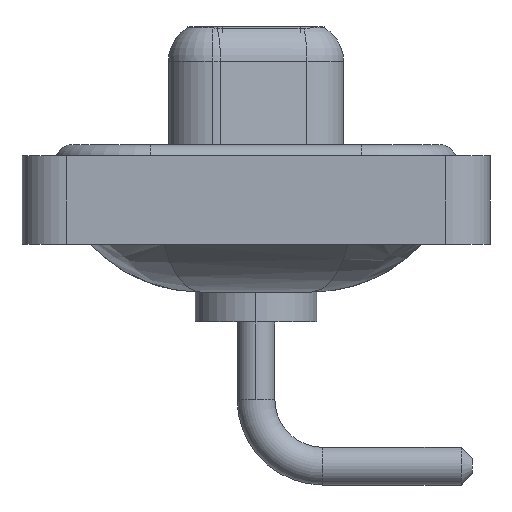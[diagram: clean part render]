
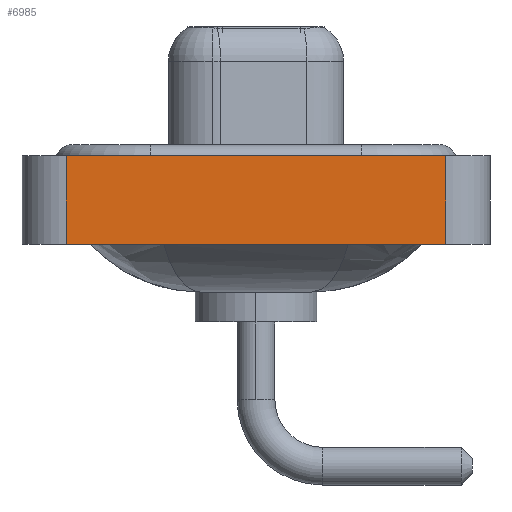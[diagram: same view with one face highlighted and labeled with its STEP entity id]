
A CAD part, left-side view. The second image highlights one B-rep face of the part: STEP entity #6985.
In plain terms, the highlighted planar face has unit normal (-1, 0, 0).
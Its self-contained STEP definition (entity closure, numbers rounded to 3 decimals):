
#455 = DIRECTION ( 'NONE',  ( -1., 0., 0. ) ) ;
#677 = DIRECTION ( 'NONE',  ( 0., 0., 1. ) ) ;
#883 = CARTESIAN_POINT ( 'NONE',  ( -7.35, -8.55, 0.4 ) ) ;
#929 = EDGE_CURVE ( 'NONE', #3650, #13558, #8184, .T. ) ;
#1572 = VECTOR ( 'NONE', #677, 1000. ) ;
#2040 = DIRECTION ( 'NONE',  ( 0., -1., 0. ) ) ;
#2259 = CARTESIAN_POINT ( 'NONE',  ( -7.35, 8.55, -3.6 ) ) ;
#2482 = VECTOR ( 'NONE', #4944, 1000. ) ;
#2557 = CARTESIAN_POINT ( 'NONE',  ( -7.35, -8.55, -3.6 ) ) ;
#3650 = VERTEX_POINT ( 'NONE', #2557 ) ;
#3830 = DIRECTION ( 'NONE',  ( 0., 0., 1. ) ) ;
#3945 = LINE ( 'NONE', #15296, #2482 ) ;
#3960 = EDGE_CURVE ( 'NONE', #14364, #13558, #15968, .T. ) ;
#4119 = FACE_OUTER_BOUND ( 'NONE', #5282, .T. ) ;
#4243 = ORIENTED_EDGE ( 'NONE', *, *, #3960, .F. ) ;
#4769 = CARTESIAN_POINT ( 'NONE',  ( -7.35, 8.55, 0.4 ) ) ;
#4944 = DIRECTION ( 'NONE',  ( 0., -1., 0. ) ) ;
#5282 = EDGE_LOOP ( 'NONE', ( #14618, #4243, #8361, #5909 ) ) ;
#5777 = EDGE_CURVE ( 'NONE', #14099, #14364, #8770, .T. ) ;
#5909 = ORIENTED_EDGE ( 'NONE', *, *, #7642, .T. ) ;
#6568 = VECTOR ( 'NONE', #2040, 1000. ) ;
#6985 = ADVANCED_FACE ( 'NONE', ( #4119 ), #15634, .T. ) ;
#7642 = EDGE_CURVE ( 'NONE', #14099, #3650, #3945, .T. ) ;
#7702 = AXIS2_PLACEMENT_3D ( 'NONE', #14469, #455, #8053 ) ;
#8053 = DIRECTION ( 'NONE',  ( 0., 0., 1. ) ) ;
#8184 = LINE ( 'NONE', #13274, #1572 ) ;
#8291 = CARTESIAN_POINT ( 'NONE',  ( -7.35, 8.55, -3.6 ) ) ;
#8361 = ORIENTED_EDGE ( 'NONE', *, *, #5777, .F. ) ;
#8770 = LINE ( 'NONE', #2259, #15095 ) ;
#12986 = CARTESIAN_POINT ( 'NONE',  ( -7.35, -8.55, 0.4 ) ) ;
#13274 = CARTESIAN_POINT ( 'NONE',  ( -7.35, -8.55, -3.6 ) ) ;
#13558 = VERTEX_POINT ( 'NONE', #12986 ) ;
#14099 = VERTEX_POINT ( 'NONE', #8291 ) ;
#14364 = VERTEX_POINT ( 'NONE', #4769 ) ;
#14469 = CARTESIAN_POINT ( 'NONE',  ( -7.35, -8.55, -3.6 ) ) ;
#14618 = ORIENTED_EDGE ( 'NONE', *, *, #929, .T. ) ;
#15095 = VECTOR ( 'NONE', #3830, 1000. ) ;
#15296 = CARTESIAN_POINT ( 'NONE',  ( -7.35, -8.55, -3.6 ) ) ;
#15634 = PLANE ( 'NONE',  #7702 ) ;
#15968 = LINE ( 'NONE', #883, #6568 ) ;
